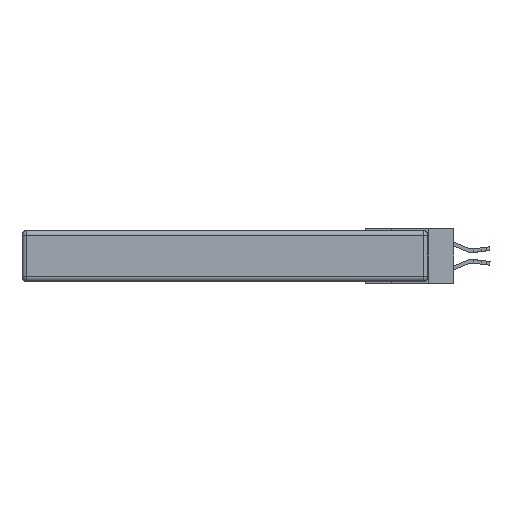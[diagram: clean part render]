
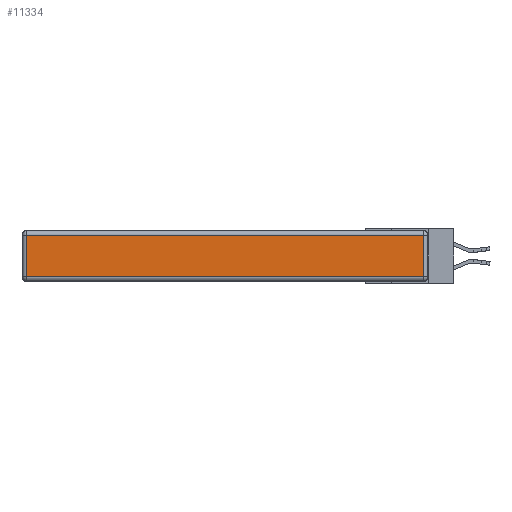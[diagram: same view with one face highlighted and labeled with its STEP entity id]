
A CAD part, left-side view. The second image highlights one B-rep face of the part: STEP entity #11334.
In plain terms, the highlighted planar face has unit normal (-1, 0, 0).
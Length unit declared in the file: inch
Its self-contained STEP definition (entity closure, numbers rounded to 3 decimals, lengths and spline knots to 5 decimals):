
#356 = CARTESIAN_POINT ( 'NONE',  ( 0., 2.72, -0.03 ) ) ;
#860 = AXIS2_PLACEMENT_3D ( 'NONE', #7359, #20512, #20589 ) ;
#1213 = CARTESIAN_POINT ( 'NONE',  ( 0., 2.75, -0.03 ) ) ;
#1297 = VECTOR ( 'NONE', #9091, 39.37008 ) ;
#1550 = CARTESIAN_POINT ( 'NONE',  ( 0., 2.72, -0.343 ) ) ;
#3005 = VERTEX_POINT ( 'NONE', #19590 ) ;
#4220 = ORIENTED_EDGE ( 'NONE', *, *, #22170, .T. ) ;
#5716 = FACE_OUTER_BOUND ( 'NONE', #22169, .T. ) ;
#5796 = LINE ( 'NONE', #12910, #11613 ) ;
#7013 = VERTEX_POINT ( 'NONE', #10863 ) ;
#7044 = EDGE_CURVE ( 'NONE', #7623, #7013, #14996, .T. ) ;
#7359 = CARTESIAN_POINT ( 'NONE',  ( 0., 0., -0.343 ) ) ;
#7623 = VERTEX_POINT ( 'NONE', #356 ) ;
#7709 = ORIENTED_EDGE ( 'NONE', *, *, #20209, .T. ) ;
#7956 = VECTOR ( 'NONE', #10624, 39.37008 ) ;
#8674 = ORIENTED_EDGE ( 'NONE', *, *, #17065, .T. ) ;
#9091 = DIRECTION ( 'NONE',  ( 0., 0., -1. ) ) ;
#10118 = CARTESIAN_POINT ( 'NONE',  ( 0., 0.03, -0.343 ) ) ;
#10624 = DIRECTION ( 'NONE',  ( 0., 1., 0. ) ) ;
#10863 = CARTESIAN_POINT ( 'NONE',  ( 0., 2.72, -0.313 ) ) ;
#11334 = ADVANCED_FACE ( 'NONE', ( #5716 ), #16843, .T. ) ;
#11613 = VECTOR ( 'NONE', #22040, 39.37008 ) ;
#12910 = CARTESIAN_POINT ( 'NONE',  ( 0., 0., -0.313 ) ) ;
#13181 = CARTESIAN_POINT ( 'NONE',  ( 0., 0.03, -0.03 ) ) ;
#13247 = LINE ( 'NONE', #1213, #7956 ) ;
#13977 = ORIENTED_EDGE ( 'NONE', *, *, #7044, .T. ) ;
#14996 = LINE ( 'NONE', #1550, #1297 ) ;
#15202 = VERTEX_POINT ( 'NONE', #13181 ) ;
#16749 = VECTOR ( 'NONE', #22057, 39.37008 ) ;
#16843 = PLANE ( 'NONE',  #860 ) ;
#17065 = EDGE_CURVE ( 'NONE', #7013, #3005, #5796, .T. ) ;
#19590 = CARTESIAN_POINT ( 'NONE',  ( 0., 0.03, -0.313 ) ) ;
#20209 = EDGE_CURVE ( 'NONE', #3005, #15202, #21691, .T. ) ;
#20512 = DIRECTION ( 'NONE',  ( -1., 0., 0. ) ) ;
#20589 = DIRECTION ( 'NONE',  ( 0., 0., 1. ) ) ;
#21691 = LINE ( 'NONE', #10118, #16749 ) ;
#22040 = DIRECTION ( 'NONE',  ( 0., -1., 0. ) ) ;
#22057 = DIRECTION ( 'NONE',  ( 0., 0., 1. ) ) ;
#22169 = EDGE_LOOP ( 'NONE', ( #8674, #7709, #4220, #13977 ) ) ;
#22170 = EDGE_CURVE ( 'NONE', #15202, #7623, #13247, .T. ) ;
